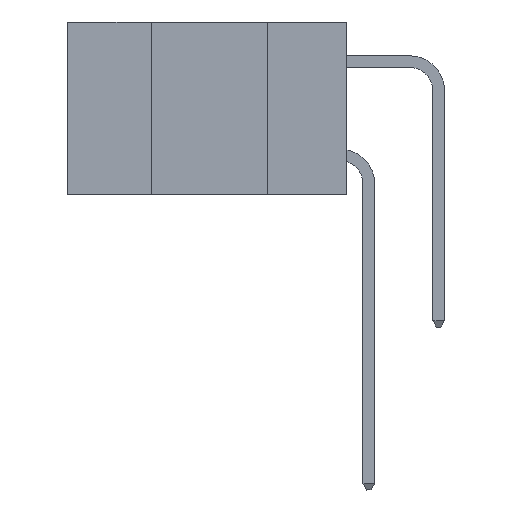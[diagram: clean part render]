
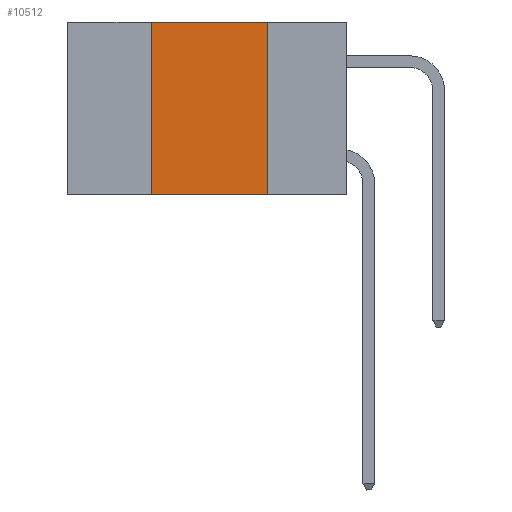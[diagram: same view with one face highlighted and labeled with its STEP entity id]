
A CAD part, left-side view. The second image highlights one B-rep face of the part: STEP entity #10512.
In plain terms, the highlighted planar face has unit normal (-1, 0, 0).
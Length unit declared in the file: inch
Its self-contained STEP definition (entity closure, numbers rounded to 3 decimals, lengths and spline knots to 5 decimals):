
#1624 = CARTESIAN_POINT ( 'NONE',  ( 0., 0.17, -0.37 ) ) ;
#2203 = CARTESIAN_POINT ( 'NONE',  ( 0., 0.17, 0. ) ) ;
#3296 = VERTEX_POINT ( 'NONE', #7656 ) ;
#4257 = LINE ( 'NONE', #11076, #7287 ) ;
#4473 = ORIENTED_EDGE ( 'NONE', *, *, #19916, .F. ) ;
#6237 = EDGE_CURVE ( 'NONE', #22186, #25269, #26849, .T. ) ;
#7287 = VECTOR ( 'NONE', #10770, 39.37008 ) ;
#7365 = DIRECTION ( 'NONE',  ( 0., 0., -1. ) ) ;
#7656 = CARTESIAN_POINT ( 'NONE',  ( 0., 0.42, -0.37 ) ) ;
#8281 = DIRECTION ( 'NONE',  ( 1., 0., 0. ) ) ;
#8419 = CARTESIAN_POINT ( 'NONE',  ( 0., 0.6, 0. ) ) ;
#8874 = VECTOR ( 'NONE', #27041, 39.37008 ) ;
#9133 = ORIENTED_EDGE ( 'NONE', *, *, #27455, .T. ) ;
#9431 = AXIS2_PLACEMENT_3D ( 'NONE', #8419, #8281, #17522 ) ;
#10512 = ADVANCED_FACE ( 'NONE', ( #29091 ), #15525, .F. ) ;
#10770 = DIRECTION ( 'NONE',  ( 0., 0., 1. ) ) ;
#11076 = CARTESIAN_POINT ( 'NONE',  ( 0., 0.42, 0. ) ) ;
#12580 = VECTOR ( 'NONE', #26702, 39.37008 ) ;
#15525 = PLANE ( 'NONE',  #9431 ) ;
#15546 = CARTESIAN_POINT ( 'NONE',  ( 0., 0.17, 0. ) ) ;
#16018 = ORIENTED_EDGE ( 'NONE', *, *, #17716, .F. ) ;
#16936 = VECTOR ( 'NONE', #7365, 39.37008 ) ;
#17337 = CARTESIAN_POINT ( 'NONE',  ( 0., 0.6, -0.37 ) ) ;
#17522 = DIRECTION ( 'NONE',  ( 0., 0., -1. ) ) ;
#17716 = EDGE_CURVE ( 'NONE', #25269, #24066, #25873, .T. ) ;
#19916 = EDGE_CURVE ( 'NONE', #3296, #22186, #4257, .T. ) ;
#20390 = ORIENTED_EDGE ( 'NONE', *, *, #6237, .F. ) ;
#22015 = CARTESIAN_POINT ( 'NONE',  ( 0., 0.6, 0. ) ) ;
#22055 = LINE ( 'NONE', #17337, #8874 ) ;
#22186 = VERTEX_POINT ( 'NONE', #24722 ) ;
#24066 = VERTEX_POINT ( 'NONE', #1624 ) ;
#24722 = CARTESIAN_POINT ( 'NONE',  ( 0., 0.42, 0. ) ) ;
#24903 = EDGE_LOOP ( 'NONE', ( #16018, #20390, #4473, #9133 ) ) ;
#25269 = VERTEX_POINT ( 'NONE', #15546 ) ;
#25873 = LINE ( 'NONE', #2203, #16936 ) ;
#26702 = DIRECTION ( 'NONE',  ( 0., -1., 0. ) ) ;
#26849 = LINE ( 'NONE', #22015, #12580 ) ;
#27041 = DIRECTION ( 'NONE',  ( 0., -1., 0. ) ) ;
#27455 = EDGE_CURVE ( 'NONE', #3296, #24066, #22055, .T. ) ;
#29091 = FACE_OUTER_BOUND ( 'NONE', #24903, .T. ) ;
